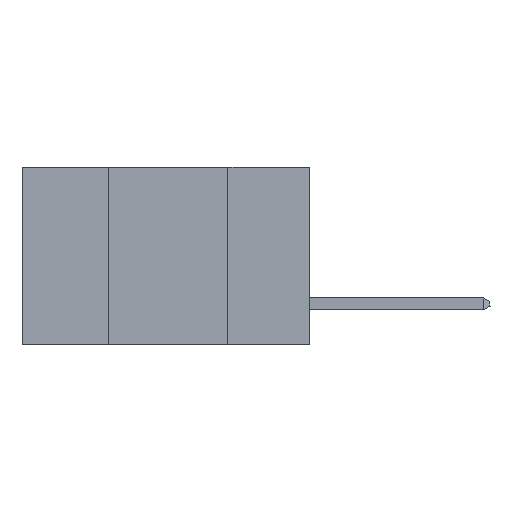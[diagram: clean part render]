
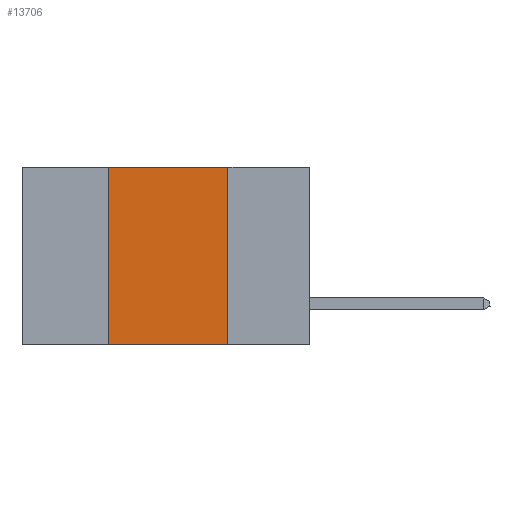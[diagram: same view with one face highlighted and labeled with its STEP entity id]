
A CAD part, left-side view. The second image highlights one B-rep face of the part: STEP entity #13706.
In plain terms, the highlighted planar face has unit normal (-1, 0, 0).
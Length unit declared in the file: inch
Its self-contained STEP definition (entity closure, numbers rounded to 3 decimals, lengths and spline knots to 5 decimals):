
#179 = DIRECTION ( 'NONE',  ( 0., -1., 0. ) ) ;
#701 = EDGE_CURVE ( 'NONE', #12887, #756, #21410, .T. ) ;
#756 = VERTEX_POINT ( 'NONE', #14851 ) ;
#892 = DIRECTION ( 'NONE',  ( 0., 0., -1. ) ) ;
#1090 = CARTESIAN_POINT ( 'NONE',  ( 0., 0.6, 0. ) ) ;
#2637 = CARTESIAN_POINT ( 'NONE',  ( 0., 0.42, 0. ) ) ;
#3016 = CARTESIAN_POINT ( 'NONE',  ( 0., 0.42, 0. ) ) ;
#3505 = VECTOR ( 'NONE', #23166, 39.37008 ) ;
#3706 = LINE ( 'NONE', #16792, #14361 ) ;
#3843 = ORIENTED_EDGE ( 'NONE', *, *, #22032, .F. ) ;
#3988 = ORIENTED_EDGE ( 'NONE', *, *, #701, .T. ) ;
#4936 = EDGE_CURVE ( 'NONE', #22877, #756, #3706, .T. ) ;
#5262 = VERTEX_POINT ( 'NONE', #2637 ) ;
#5386 = AXIS2_PLACEMENT_3D ( 'NONE', #20518, #17072, #892 ) ;
#7215 = CARTESIAN_POINT ( 'NONE',  ( 0., 0.17, 0. ) ) ;
#7830 = ORIENTED_EDGE ( 'NONE', *, *, #13300, .F. ) ;
#10060 = DIRECTION ( 'NONE',  ( 0., -1., 0. ) ) ;
#11398 = EDGE_LOOP ( 'NONE', ( #23163, #7830, #3843, #3988 ) ) ;
#12887 = VERTEX_POINT ( 'NONE', #20253 ) ;
#13300 = EDGE_CURVE ( 'NONE', #5262, #22877, #14084, .T. ) ;
#13368 = DIRECTION ( 'NONE',  ( 0., 0., -1. ) ) ;
#13706 = ADVANCED_FACE ( 'NONE', ( #15776 ), #18674, .F. ) ;
#14084 = LINE ( 'NONE', #1090, #15958 ) ;
#14361 = VECTOR ( 'NONE', #13368, 39.37008 ) ;
#14851 = CARTESIAN_POINT ( 'NONE',  ( 0., 0.17, -0.37 ) ) ;
#15776 = FACE_OUTER_BOUND ( 'NONE', #11398, .T. ) ;
#15958 = VECTOR ( 'NONE', #10060, 39.37008 ) ;
#16410 = LINE ( 'NONE', #3016, #3505 ) ;
#16792 = CARTESIAN_POINT ( 'NONE',  ( 0., 0.17, 0. ) ) ;
#16822 = CARTESIAN_POINT ( 'NONE',  ( 0., 0.6, -0.37 ) ) ;
#17072 = DIRECTION ( 'NONE',  ( 1., 0., 0. ) ) ;
#18674 = PLANE ( 'NONE',  #5386 ) ;
#20253 = CARTESIAN_POINT ( 'NONE',  ( 0., 0.42, -0.37 ) ) ;
#20518 = CARTESIAN_POINT ( 'NONE',  ( 0., 0.6, 0. ) ) ;
#21410 = LINE ( 'NONE', #16822, #22562 ) ;
#22032 = EDGE_CURVE ( 'NONE', #12887, #5262, #16410, .T. ) ;
#22562 = VECTOR ( 'NONE', #179, 39.37008 ) ;
#22877 = VERTEX_POINT ( 'NONE', #7215 ) ;
#23163 = ORIENTED_EDGE ( 'NONE', *, *, #4936, .F. ) ;
#23166 = DIRECTION ( 'NONE',  ( 0., 0., 1. ) ) ;
